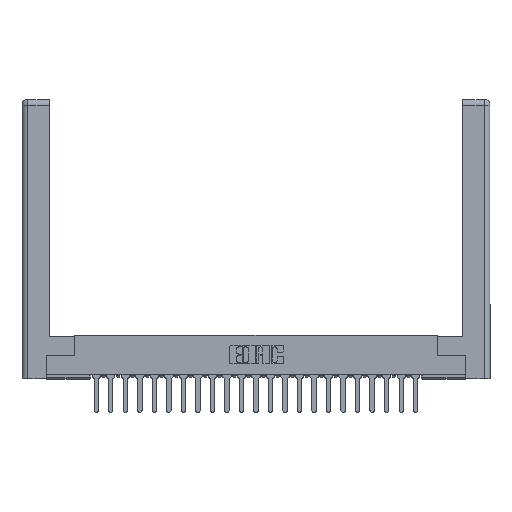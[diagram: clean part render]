
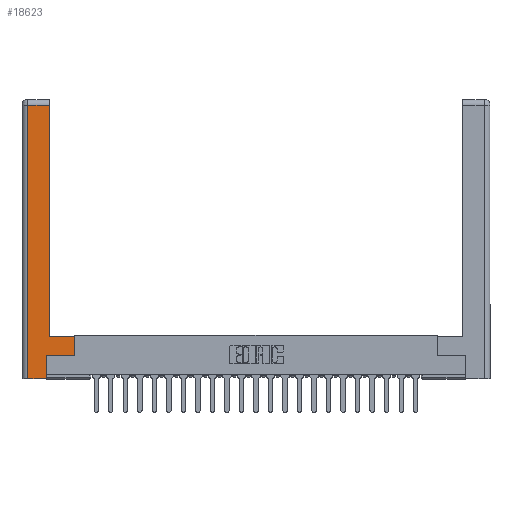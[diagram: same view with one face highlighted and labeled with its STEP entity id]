
A CAD part, top view. The second image highlights one B-rep face of the part: STEP entity #18623.
In plain terms, the highlighted planar face has unit normal (0, 0, 1).
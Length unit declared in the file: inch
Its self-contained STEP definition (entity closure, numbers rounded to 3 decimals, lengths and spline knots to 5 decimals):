
#361 = LINE ( 'NONE', #6060, #3421 ) ;
#944 = EDGE_CURVE ( 'NONE', #3723, #17557, #22766, .T. ) ;
#1419 = ORIENTED_EDGE ( 'NONE', *, *, #2449, .T. ) ;
#1497 = LINE ( 'NONE', #9106, #17691 ) ;
#1667 = VERTEX_POINT ( 'NONE', #5292 ) ;
#1748 = VECTOR ( 'NONE', #15200, 39.37008 ) ;
#1780 = FACE_OUTER_BOUND ( 'NONE', #8872, .T. ) ;
#2449 = EDGE_CURVE ( 'NONE', #23874, #8798, #18076, .T. ) ;
#3052 = PLANE ( 'NONE',  #12143 ) ;
#3421 = VECTOR ( 'NONE', #9581, 39.37008 ) ;
#3723 = VERTEX_POINT ( 'NONE', #15059 ) ;
#4012 = DIRECTION ( 'NONE',  ( 0., 1., 0. ) ) ;
#4462 = LINE ( 'NONE', #19605, #7382 ) ;
#5045 = ORIENTED_EDGE ( 'NONE', *, *, #19661, .T. ) ;
#5292 = CARTESIAN_POINT ( 'NONE',  ( 0.295, 0.45, 0. ) ) ;
#5860 = EDGE_CURVE ( 'NONE', #17557, #10769, #17766, .T. ) ;
#6060 = CARTESIAN_POINT ( 'NONE',  ( 0.0615, 0., 0. ) ) ;
#6327 = CARTESIAN_POINT ( 'NONE',  ( 0.0615, 0., 0. ) ) ;
#6493 = EDGE_CURVE ( 'NONE', #10769, #13500, #1497, .T. ) ;
#6925 = CARTESIAN_POINT ( 'NONE',  ( 0., 0., 0. ) ) ;
#7382 = VECTOR ( 'NONE', #21972, 39.37008 ) ;
#7628 = ORIENTED_EDGE ( 'NONE', *, *, #12435, .T. ) ;
#7828 = VECTOR ( 'NONE', #18087, 39.37008 ) ;
#7849 = CARTESIAN_POINT ( 'NONE',  ( 0.295, 0.45, 0. ) ) ;
#8591 = CARTESIAN_POINT ( 'NONE',  ( 0.295, 3., 0. ) ) ;
#8707 = DIRECTION ( 'NONE',  ( -1., 0., 0. ) ) ;
#8798 = VERTEX_POINT ( 'NONE', #18234 ) ;
#8801 = DIRECTION ( 'NONE',  ( -1., 0., 0. ) ) ;
#8872 = EDGE_LOOP ( 'NONE', ( #13826, #1419, #5045, #7628, #18857, #14057, #21269, #10923 ) ) ;
#9106 = CARTESIAN_POINT ( 'NONE',  ( 0.565, 0.45, 0. ) ) ;
#9581 = DIRECTION ( 'NONE',  ( 0., -1., 0. ) ) ;
#10001 = DIRECTION ( 'NONE',  ( 1., 0., 0. ) ) ;
#10435 = CARTESIAN_POINT ( 'NONE',  ( 0.0615, 2.94, 0. ) ) ;
#10769 = VERTEX_POINT ( 'NONE', #23384 ) ;
#10923 = ORIENTED_EDGE ( 'NONE', *, *, #12762, .T. ) ;
#12143 = AXIS2_PLACEMENT_3D ( 'NONE', #6925, #14658, #8801 ) ;
#12435 = EDGE_CURVE ( 'NONE', #12834, #3723, #4462, .T. ) ;
#12762 = EDGE_CURVE ( 'NONE', #13500, #1667, #16972, .T. ) ;
#12834 = VERTEX_POINT ( 'NONE', #6327 ) ;
#13500 = VERTEX_POINT ( 'NONE', #14653 ) ;
#13826 = ORIENTED_EDGE ( 'NONE', *, *, #15249, .T. ) ;
#14057 = ORIENTED_EDGE ( 'NONE', *, *, #5860, .T. ) ;
#14230 = CARTESIAN_POINT ( 'NONE',  ( 0.565, 0.245, 0. ) ) ;
#14653 = CARTESIAN_POINT ( 'NONE',  ( 0.565, 0.45, 0. ) ) ;
#14658 = DIRECTION ( 'NONE',  ( 0., 0., -1. ) ) ;
#15059 = CARTESIAN_POINT ( 'NONE',  ( 0.265, 0., 0. ) ) ;
#15200 = DIRECTION ( 'NONE',  ( -1., 0., 0. ) ) ;
#15249 = EDGE_CURVE ( 'NONE', #1667, #23874, #21588, .T. ) ;
#16972 = LINE ( 'NONE', #7849, #1748 ) ;
#17248 = CARTESIAN_POINT ( 'NONE',  ( 0.295, 2.94, 0. ) ) ;
#17557 = VERTEX_POINT ( 'NONE', #18288 ) ;
#17650 = VECTOR ( 'NONE', #10001, 39.37008 ) ;
#17691 = VECTOR ( 'NONE', #18730, 39.37008 ) ;
#17766 = LINE ( 'NONE', #14230, #17650 ) ;
#18076 = LINE ( 'NONE', #10435, #23206 ) ;
#18087 = DIRECTION ( 'NONE',  ( 0., 1., 0. ) ) ;
#18234 = CARTESIAN_POINT ( 'NONE',  ( 0.0615, 2.94, 0. ) ) ;
#18288 = CARTESIAN_POINT ( 'NONE',  ( 0.265, 0.245, 0. ) ) ;
#18623 = ADVANCED_FACE ( 'NONE', ( #1780 ), #3052, .F. ) ;
#18730 = DIRECTION ( 'NONE',  ( 0., 1., 0. ) ) ;
#18857 = ORIENTED_EDGE ( 'NONE', *, *, #944, .T. ) ;
#19155 = CARTESIAN_POINT ( 'NONE',  ( 0.265, 0.245, 0. ) ) ;
#19605 = CARTESIAN_POINT ( 'NONE',  ( 0.265, 0., 0. ) ) ;
#19661 = EDGE_CURVE ( 'NONE', #8798, #12834, #361, .T. ) ;
#20268 = VECTOR ( 'NONE', #4012, 39.37008 ) ;
#21269 = ORIENTED_EDGE ( 'NONE', *, *, #6493, .T. ) ;
#21588 = LINE ( 'NONE', #8591, #7828 ) ;
#21972 = DIRECTION ( 'NONE',  ( 1., 0., 0. ) ) ;
#22766 = LINE ( 'NONE', #19155, #20268 ) ;
#23206 = VECTOR ( 'NONE', #8707, 39.37008 ) ;
#23384 = CARTESIAN_POINT ( 'NONE',  ( 0.565, 0.245, 0. ) ) ;
#23874 = VERTEX_POINT ( 'NONE', #17248 ) ;
